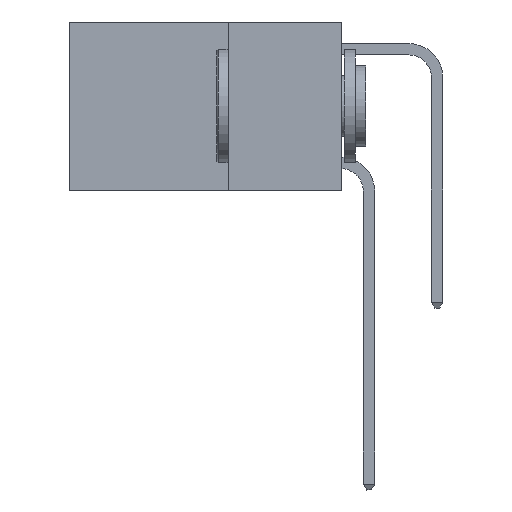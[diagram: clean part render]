
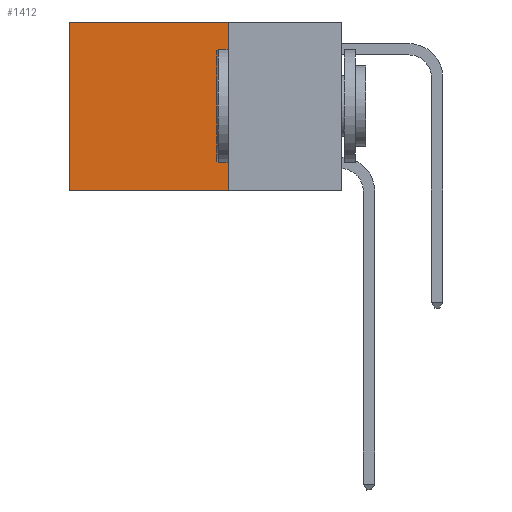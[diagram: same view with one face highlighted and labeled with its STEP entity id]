
A CAD part, left-side view. The second image highlights one B-rep face of the part: STEP entity #1412.
In plain terms, the highlighted planar face has unit normal (-1, 0, 0).
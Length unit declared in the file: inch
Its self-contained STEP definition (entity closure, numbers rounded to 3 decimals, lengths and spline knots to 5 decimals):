
#33 = VECTOR ( 'NONE', #18315, 39.37008 ) ;
#370 = CARTESIAN_POINT ( 'NONE',  ( 0.2625, 0.25, 0. ) ) ;
#428 = CARTESIAN_POINT ( 'NONE',  ( 0.2625, 0.25, 0. ) ) ;
#1412 = ADVANCED_FACE ( 'NONE', ( #8865 ), #11466, .F. ) ;
#1452 = DIRECTION ( 'NONE',  ( 0., 0., -1. ) ) ;
#1541 = CARTESIAN_POINT ( 'NONE',  ( 0.2625, 0.25, 0. ) ) ;
#1702 = CARTESIAN_POINT ( 'NONE',  ( 0.2625, 0.6, -0.37 ) ) ;
#3652 = AXIS2_PLACEMENT_3D ( 'NONE', #370, #6064, #4690 ) ;
#3819 = LINE ( 'NONE', #17651, #15336 ) ;
#4538 = DIRECTION ( 'NONE',  ( 0., 1., 0. ) ) ;
#4690 = DIRECTION ( 'NONE',  ( 0., 0., -1. ) ) ;
#5729 = VERTEX_POINT ( 'NONE', #9404 ) ;
#6064 = DIRECTION ( 'NONE',  ( 1., 0., 0. ) ) ;
#6169 = VERTEX_POINT ( 'NONE', #17829 ) ;
#6524 = EDGE_CURVE ( 'NONE', #5729, #9208, #9919, .T. ) ;
#7848 = LINE ( 'NONE', #11075, #33 ) ;
#8569 = EDGE_CURVE ( 'NONE', #17590, #5729, #17074, .T. ) ;
#8812 = ORIENTED_EDGE ( 'NONE', *, *, #14382, .T. ) ;
#8865 = FACE_OUTER_BOUND ( 'NONE', #16185, .T. ) ;
#9208 = VERTEX_POINT ( 'NONE', #1702 ) ;
#9258 = EDGE_CURVE ( 'NONE', #17590, #6169, #7848, .T. ) ;
#9404 = CARTESIAN_POINT ( 'NONE',  ( 0.2625, 0.25, -0.37 ) ) ;
#9547 = VECTOR ( 'NONE', #1452, 39.37008 ) ;
#9919 = LINE ( 'NONE', #15757, #14873 ) ;
#11075 = CARTESIAN_POINT ( 'NONE',  ( 0.2625, 0.25, 0. ) ) ;
#11466 = PLANE ( 'NONE',  #3652 ) ;
#13353 = ORIENTED_EDGE ( 'NONE', *, *, #8569, .F. ) ;
#13762 = ORIENTED_EDGE ( 'NONE', *, *, #6524, .F. ) ;
#14382 = EDGE_CURVE ( 'NONE', #6169, #9208, #3819, .T. ) ;
#14873 = VECTOR ( 'NONE', #4538, 39.37008 ) ;
#15336 = VECTOR ( 'NONE', #16260, 39.37008 ) ;
#15757 = CARTESIAN_POINT ( 'NONE',  ( 0.2625, 0.25, -0.37 ) ) ;
#16185 = EDGE_LOOP ( 'NONE', ( #8812, #13762, #13353, #16201 ) ) ;
#16201 = ORIENTED_EDGE ( 'NONE', *, *, #9258, .T. ) ;
#16260 = DIRECTION ( 'NONE',  ( 0., 0., -1. ) ) ;
#17074 = LINE ( 'NONE', #1541, #9547 ) ;
#17590 = VERTEX_POINT ( 'NONE', #428 ) ;
#17651 = CARTESIAN_POINT ( 'NONE',  ( 0.2625, 0.6, 0. ) ) ;
#17829 = CARTESIAN_POINT ( 'NONE',  ( 0.2625, 0.6, 0. ) ) ;
#18315 = DIRECTION ( 'NONE',  ( 0., 1., 0. ) ) ;
